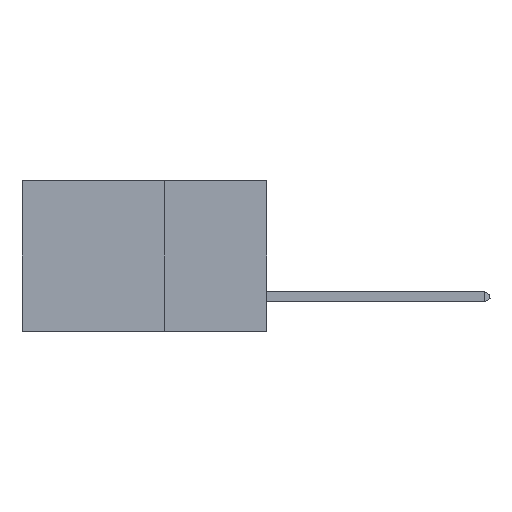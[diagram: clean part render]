
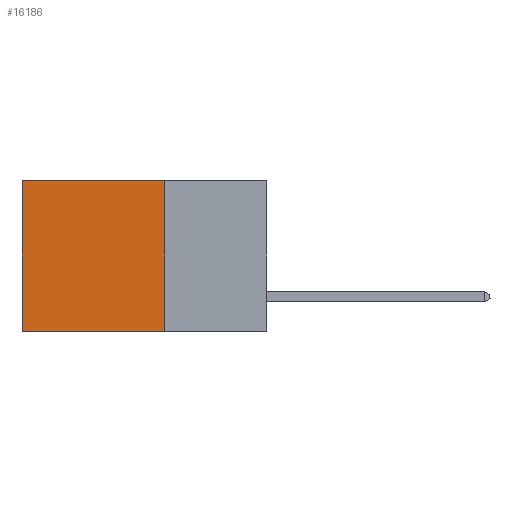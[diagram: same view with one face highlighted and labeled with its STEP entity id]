
A CAD part, left-side view. The second image highlights one B-rep face of the part: STEP entity #16186.
In plain terms, the highlighted planar face has unit normal (-1, 0, 0).
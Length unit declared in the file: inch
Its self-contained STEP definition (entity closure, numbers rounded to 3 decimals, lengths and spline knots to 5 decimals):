
#137 = VERTEX_POINT ( 'NONE', #14350 ) ;
#1491 = DIRECTION ( 'NONE',  ( 0., 1., 0. ) ) ;
#1539 = ORIENTED_EDGE ( 'NONE', *, *, #15433, .T. ) ;
#1810 = VERTEX_POINT ( 'NONE', #17861 ) ;
#2038 = CARTESIAN_POINT ( 'NONE',  ( 0.2875, 0.6, -0.37 ) ) ;
#2631 = VECTOR ( 'NONE', #10229, 39.37008 ) ;
#3734 = ORIENTED_EDGE ( 'NONE', *, *, #14694, .F. ) ;
#3919 = LINE ( 'NONE', #6835, #2631 ) ;
#5336 = DIRECTION ( 'NONE',  ( 1., 0., 0. ) ) ;
#5432 = ORIENTED_EDGE ( 'NONE', *, *, #6980, .F. ) ;
#6039 = VECTOR ( 'NONE', #6400, 39.37008 ) ;
#6400 = DIRECTION ( 'NONE',  ( 0., 1., 0. ) ) ;
#6610 = DIRECTION ( 'NONE',  ( 0., 0., -1. ) ) ;
#6835 = CARTESIAN_POINT ( 'NONE',  ( 0.2875, 0.6, 0. ) ) ;
#6980 = EDGE_CURVE ( 'NONE', #137, #10568, #21013, .T. ) ;
#8629 = LINE ( 'NONE', #18280, #10910 ) ;
#9201 = ORIENTED_EDGE ( 'NONE', *, *, #12244, .T. ) ;
#9883 = FACE_OUTER_BOUND ( 'NONE', #11448, .T. ) ;
#10229 = DIRECTION ( 'NONE',  ( 0., 0., -1. ) ) ;
#10568 = VERTEX_POINT ( 'NONE', #2038 ) ;
#10619 = AXIS2_PLACEMENT_3D ( 'NONE', #20016, #5336, #16751 ) ;
#10910 = VECTOR ( 'NONE', #6610, 39.37008 ) ;
#11232 = CARTESIAN_POINT ( 'NONE',  ( 0.2875, 0.25, -0.37 ) ) ;
#11300 = CARTESIAN_POINT ( 'NONE',  ( 0.2875, 0.6, 0. ) ) ;
#11448 = EDGE_LOOP ( 'NONE', ( #9201, #5432, #3734, #1539 ) ) ;
#11605 = VECTOR ( 'NONE', #1491, 39.37008 ) ;
#11610 = VERTEX_POINT ( 'NONE', #11300 ) ;
#12244 = EDGE_CURVE ( 'NONE', #11610, #10568, #3919, .T. ) ;
#14350 = CARTESIAN_POINT ( 'NONE',  ( 0.2875, 0.25, -0.37 ) ) ;
#14694 = EDGE_CURVE ( 'NONE', #1810, #137, #8629, .T. ) ;
#15433 = EDGE_CURVE ( 'NONE', #1810, #11610, #16527, .T. ) ;
#16186 = ADVANCED_FACE ( 'NONE', ( #9883 ), #18369, .F. ) ;
#16527 = LINE ( 'NONE', #19429, #6039 ) ;
#16751 = DIRECTION ( 'NONE',  ( 0., 0., -1. ) ) ;
#17861 = CARTESIAN_POINT ( 'NONE',  ( 0.2875, 0.25, 0. ) ) ;
#18280 = CARTESIAN_POINT ( 'NONE',  ( 0.2875, 0.25, 0. ) ) ;
#18369 = PLANE ( 'NONE',  #10619 ) ;
#19429 = CARTESIAN_POINT ( 'NONE',  ( 0.2875, 0.25, 0. ) ) ;
#20016 = CARTESIAN_POINT ( 'NONE',  ( 0.2875, 0.25, 0. ) ) ;
#21013 = LINE ( 'NONE', #11232, #11605 ) ;
